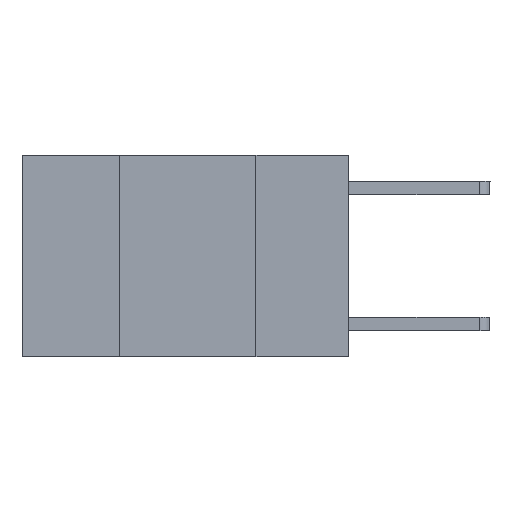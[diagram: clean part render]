
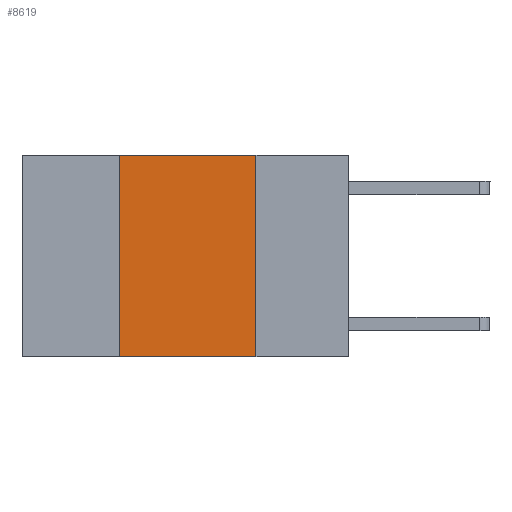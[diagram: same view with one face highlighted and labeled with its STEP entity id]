
A CAD part, left-side view. The second image highlights one B-rep face of the part: STEP entity #8619.
In plain terms, the highlighted planar face has unit normal (-1, 0, 0).
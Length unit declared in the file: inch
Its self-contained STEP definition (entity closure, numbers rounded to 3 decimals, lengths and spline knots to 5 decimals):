
#113 = CARTESIAN_POINT ( 'NONE',  ( 0., 0.6, -0.37 ) ) ;
#187 = LINE ( 'NONE', #6447, #7595 ) ;
#225 = ORIENTED_EDGE ( 'NONE', *, *, #2842, .F. ) ;
#495 = ORIENTED_EDGE ( 'NONE', *, *, #1267, .F. ) ;
#537 = VECTOR ( 'NONE', #4936, 39.37008 ) ;
#639 = VECTOR ( 'NONE', #1348, 39.37008 ) ;
#770 = LINE ( 'NONE', #7417, #537 ) ;
#1003 = CARTESIAN_POINT ( 'NONE',  ( 0., 0.17, -0.37 ) ) ;
#1223 = VERTEX_POINT ( 'NONE', #1003 ) ;
#1267 = EDGE_CURVE ( 'NONE', #5188, #1223, #770, .T. ) ;
#1300 = EDGE_CURVE ( 'NONE', #4627, #5591, #2274, .T. ) ;
#1348 = DIRECTION ( 'NONE',  ( 0., -1., 0. ) ) ;
#1477 = CARTESIAN_POINT ( 'NONE',  ( 0., 0.42, -0.37 ) ) ;
#1511 = EDGE_CURVE ( 'NONE', #4627, #1223, #6202, .T. ) ;
#2274 = LINE ( 'NONE', #5998, #3983 ) ;
#2314 = ORIENTED_EDGE ( 'NONE', *, *, #1511, .T. ) ;
#2842 = EDGE_CURVE ( 'NONE', #5591, #5188, #187, .T. ) ;
#3504 = DIRECTION ( 'NONE',  ( 1., 0., 0. ) ) ;
#3535 = ORIENTED_EDGE ( 'NONE', *, *, #1300, .F. ) ;
#3983 = VECTOR ( 'NONE', #7928, 39.37008 ) ;
#4211 = PLANE ( 'NONE',  #6407 ) ;
#4627 = VERTEX_POINT ( 'NONE', #1477 ) ;
#4936 = DIRECTION ( 'NONE',  ( 0., 0., -1. ) ) ;
#5188 = VERTEX_POINT ( 'NONE', #6955 ) ;
#5326 = CARTESIAN_POINT ( 'NONE',  ( 0., 0.42, 0. ) ) ;
#5440 = FACE_OUTER_BOUND ( 'NONE', #8244, .T. ) ;
#5591 = VERTEX_POINT ( 'NONE', #5326 ) ;
#5998 = CARTESIAN_POINT ( 'NONE',  ( 0., 0.42, 0. ) ) ;
#6202 = LINE ( 'NONE', #113, #639 ) ;
#6407 = AXIS2_PLACEMENT_3D ( 'NONE', #7698, #3504, #8387 ) ;
#6447 = CARTESIAN_POINT ( 'NONE',  ( 0., 0.6, 0. ) ) ;
#6955 = CARTESIAN_POINT ( 'NONE',  ( 0., 0.17, 0. ) ) ;
#7417 = CARTESIAN_POINT ( 'NONE',  ( 0., 0.17, 0. ) ) ;
#7595 = VECTOR ( 'NONE', #8447, 39.37008 ) ;
#7698 = CARTESIAN_POINT ( 'NONE',  ( 0., 0.6, 0. ) ) ;
#7928 = DIRECTION ( 'NONE',  ( 0., 0., 1. ) ) ;
#8244 = EDGE_LOOP ( 'NONE', ( #495, #225, #3535, #2314 ) ) ;
#8387 = DIRECTION ( 'NONE',  ( 0., 0., -1. ) ) ;
#8447 = DIRECTION ( 'NONE',  ( 0., -1., 0. ) ) ;
#8619 = ADVANCED_FACE ( 'NONE', ( #5440 ), #4211, .F. ) ;
